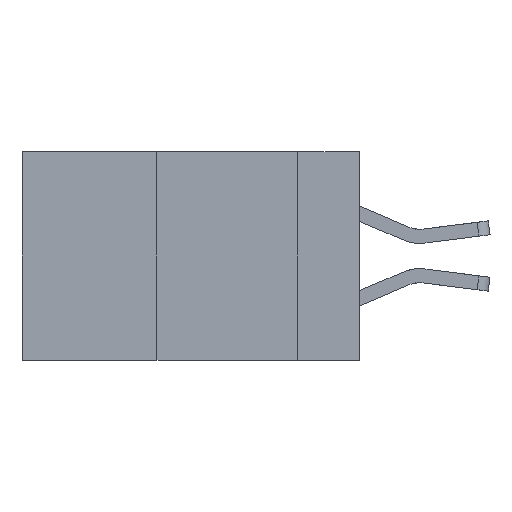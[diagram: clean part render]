
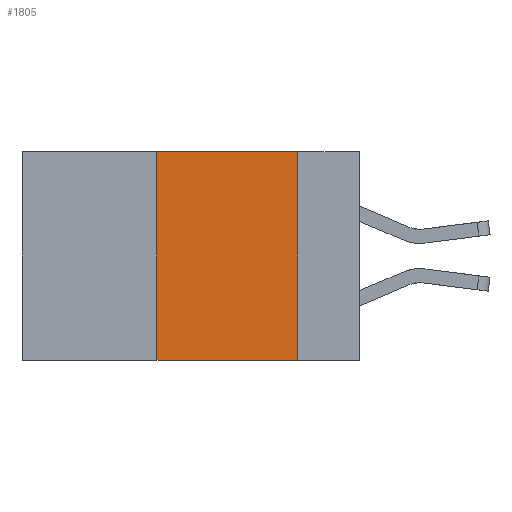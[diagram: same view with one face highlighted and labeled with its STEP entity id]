
A CAD part, left-side view. The second image highlights one B-rep face of the part: STEP entity #1805.
In plain terms, the highlighted planar face has unit normal (-1, 0, 0).
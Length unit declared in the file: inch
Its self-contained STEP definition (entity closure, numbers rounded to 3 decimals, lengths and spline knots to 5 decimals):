
#9 = AXIS2_PLACEMENT_3D ( 'NONE', #5077, #9975, #3245 ) ;
#231 = VECTOR ( 'NONE', #9575, 39.37008 ) ;
#651 = DIRECTION ( 'NONE',  ( 0., 0., 1. ) ) ;
#761 = LINE ( 'NONE', #6599, #231 ) ;
#1166 = DIRECTION ( 'NONE',  ( 0., -1., 0. ) ) ;
#1727 = CARTESIAN_POINT ( 'NONE',  ( 0., 0.11, -0.37 ) ) ;
#1805 = ADVANCED_FACE ( 'NONE', ( #8146 ), #2368, .F. ) ;
#1870 = VERTEX_POINT ( 'NONE', #1727 ) ;
#2264 = EDGE_CURVE ( 'NONE', #10766, #1870, #5247, .T. ) ;
#2280 = VECTOR ( 'NONE', #651, 39.37008 ) ;
#2336 = VERTEX_POINT ( 'NONE', #3664 ) ;
#2368 = PLANE ( 'NONE',  #9 ) ;
#2594 = CARTESIAN_POINT ( 'NONE',  ( 0., 0.36, 0. ) ) ;
#2703 = ORIENTED_EDGE ( 'NONE', *, *, #7250, .F. ) ;
#3118 = LINE ( 'NONE', #7824, #11031 ) ;
#3245 = DIRECTION ( 'NONE',  ( 0., 0., -1. ) ) ;
#3359 = DIRECTION ( 'NONE',  ( 0., 0., -1. ) ) ;
#3486 = LINE ( 'NONE', #2594, #2280 ) ;
#3664 = CARTESIAN_POINT ( 'NONE',  ( 0., 0.36, 0. ) ) ;
#4318 = CARTESIAN_POINT ( 'NONE',  ( 0., 0.11, 0. ) ) ;
#5077 = CARTESIAN_POINT ( 'NONE',  ( 0., 0.6, 0. ) ) ;
#5247 = LINE ( 'NONE', #4318, #5639 ) ;
#5639 = VECTOR ( 'NONE', #3359, 39.37008 ) ;
#6384 = ORIENTED_EDGE ( 'NONE', *, *, #11247, .T. ) ;
#6599 = CARTESIAN_POINT ( 'NONE',  ( 0., 0.6, 0. ) ) ;
#6626 = ORIENTED_EDGE ( 'NONE', *, *, #2264, .F. ) ;
#7250 = EDGE_CURVE ( 'NONE', #10546, #2336, #3486, .T. ) ;
#7824 = CARTESIAN_POINT ( 'NONE',  ( 0., 0.6, -0.37 ) ) ;
#8042 = EDGE_LOOP ( 'NONE', ( #6626, #10565, #2703, #6384 ) ) ;
#8146 = FACE_OUTER_BOUND ( 'NONE', #8042, .T. ) ;
#8550 = CARTESIAN_POINT ( 'NONE',  ( 0., 0.11, 0. ) ) ;
#9575 = DIRECTION ( 'NONE',  ( 0., -1., 0. ) ) ;
#9975 = DIRECTION ( 'NONE',  ( 1., 0., 0. ) ) ;
#10546 = VERTEX_POINT ( 'NONE', #11113 ) ;
#10565 = ORIENTED_EDGE ( 'NONE', *, *, #12229, .F. ) ;
#10766 = VERTEX_POINT ( 'NONE', #8550 ) ;
#11031 = VECTOR ( 'NONE', #1166, 39.37008 ) ;
#11113 = CARTESIAN_POINT ( 'NONE',  ( 0., 0.36, -0.37 ) ) ;
#11247 = EDGE_CURVE ( 'NONE', #10546, #1870, #3118, .T. ) ;
#12229 = EDGE_CURVE ( 'NONE', #2336, #10766, #761, .T. ) ;
